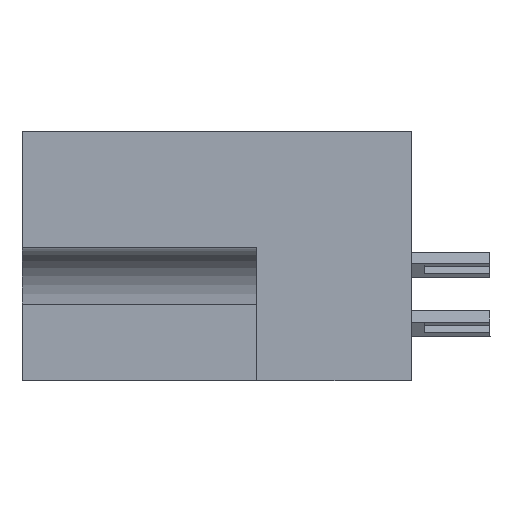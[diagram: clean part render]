
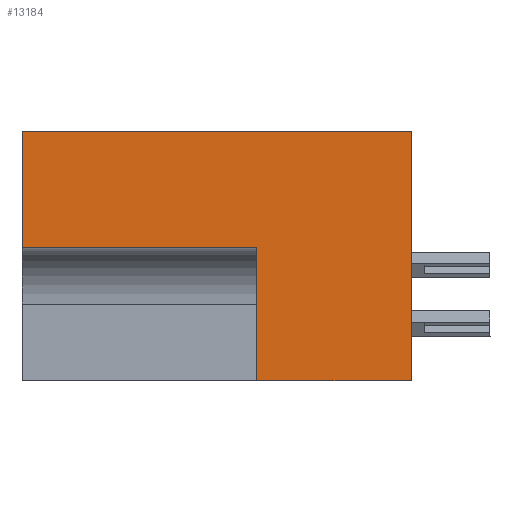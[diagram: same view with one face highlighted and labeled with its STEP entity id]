
A CAD part, left-side view. The second image highlights one B-rep face of the part: STEP entity #13184.
In plain terms, the highlighted planar face has unit normal (-1, 0, 0).
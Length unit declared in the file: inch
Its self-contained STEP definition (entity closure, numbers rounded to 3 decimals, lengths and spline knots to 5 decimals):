
#167 = DIRECTION ( 'NONE',  ( 0., 0., 1. ) ) ;
#720 = LINE ( 'NONE', #21529, #15058 ) ;
#978 = LINE ( 'NONE', #14258, #24172 ) ;
#2013 = EDGE_CURVE ( 'NONE', #28216, #18492, #19542, .T. ) ;
#3158 = CARTESIAN_POINT ( 'NONE',  ( 0., 0., 0. ) ) ;
#3529 = VERTEX_POINT ( 'NONE', #26431 ) ;
#4109 = LINE ( 'NONE', #23786, #12948 ) ;
#4532 = DIRECTION ( 'NONE',  ( 1., 0., 0. ) ) ;
#4587 = AXIS2_PLACEMENT_3D ( 'NONE', #11522, #4532, #9966 ) ;
#5033 = EDGE_CURVE ( 'NONE', #18492, #9611, #13115, .T. ) ;
#6255 = DIRECTION ( 'NONE',  ( 0., -1., 0. ) ) ;
#6435 = EDGE_LOOP ( 'NONE', ( #24551, #23287, #16511, #24964, #24989, #19899 ) ) ;
#9611 = VERTEX_POINT ( 'NONE', #28509 ) ;
#9966 = DIRECTION ( 'NONE',  ( 0., 0., -1. ) ) ;
#10061 = LINE ( 'NONE', #21940, #19622 ) ;
#10692 = VERTEX_POINT ( 'NONE', #24015 ) ;
#11098 = CARTESIAN_POINT ( 'NONE',  ( 0., 0.453, -0.531 ) ) ;
#11186 = CARTESIAN_POINT ( 'NONE',  ( 0., 0., -0.531 ) ) ;
#11245 = CARTESIAN_POINT ( 'NONE',  ( 0., 0.828, 0. ) ) ;
#11522 = CARTESIAN_POINT ( 'NONE',  ( 0., 0.453, 0. ) ) ;
#12258 = EDGE_CURVE ( 'NONE', #28198, #9611, #10061, .T. ) ;
#12635 = DIRECTION ( 'NONE',  ( 0., 0., 1. ) ) ;
#12948 = VECTOR ( 'NONE', #14121, 39.37008 ) ;
#13115 = LINE ( 'NONE', #3158, #20087 ) ;
#13184 = ADVANCED_FACE ( 'NONE', ( #28039 ), #21063, .F. ) ;
#13649 = VECTOR ( 'NONE', #6255, 39.37008 ) ;
#13837 = CARTESIAN_POINT ( 'NONE',  ( 0., 0.328, -0.531 ) ) ;
#14121 = DIRECTION ( 'NONE',  ( 0., 1., 0. ) ) ;
#14258 = CARTESIAN_POINT ( 'NONE',  ( 0., 0.828, 0. ) ) ;
#15058 = VECTOR ( 'NONE', #26176, 39.37008 ) ;
#16455 = EDGE_CURVE ( 'NONE', #10692, #28198, #978, .T. ) ;
#16511 = ORIENTED_EDGE ( 'NONE', *, *, #29806, .F. ) ;
#18492 = VERTEX_POINT ( 'NONE', #11186 ) ;
#19369 = DIRECTION ( 'NONE',  ( 0., -1., 0. ) ) ;
#19542 = LINE ( 'NONE', #11098, #13649 ) ;
#19622 = VECTOR ( 'NONE', #19369, 39.37008 ) ;
#19709 = EDGE_CURVE ( 'NONE', #3529, #10692, #4109, .T. ) ;
#19899 = ORIENTED_EDGE ( 'NONE', *, *, #12258, .F. ) ;
#20087 = VECTOR ( 'NONE', #12635, 39.37008 ) ;
#21063 = PLANE ( 'NONE',  #4587 ) ;
#21529 = CARTESIAN_POINT ( 'NONE',  ( 0., 0.328, -0.531 ) ) ;
#21940 = CARTESIAN_POINT ( 'NONE',  ( 0., 0.453, 0. ) ) ;
#23287 = ORIENTED_EDGE ( 'NONE', *, *, #19709, .F. ) ;
#23786 = CARTESIAN_POINT ( 'NONE',  ( 0., 0.328, -0.248 ) ) ;
#24015 = CARTESIAN_POINT ( 'NONE',  ( 0., 0.828, -0.248 ) ) ;
#24172 = VECTOR ( 'NONE', #167, 39.37008 ) ;
#24551 = ORIENTED_EDGE ( 'NONE', *, *, #16455, .F. ) ;
#24964 = ORIENTED_EDGE ( 'NONE', *, *, #2013, .T. ) ;
#24989 = ORIENTED_EDGE ( 'NONE', *, *, #5033, .T. ) ;
#26176 = DIRECTION ( 'NONE',  ( 0., 0., 1. ) ) ;
#26431 = CARTESIAN_POINT ( 'NONE',  ( 0., 0.328, -0.248 ) ) ;
#28039 = FACE_OUTER_BOUND ( 'NONE', #6435, .T. ) ;
#28198 = VERTEX_POINT ( 'NONE', #11245 ) ;
#28216 = VERTEX_POINT ( 'NONE', #13837 ) ;
#28509 = CARTESIAN_POINT ( 'NONE',  ( 0., 0., 0. ) ) ;
#29806 = EDGE_CURVE ( 'NONE', #28216, #3529, #720, .T. ) ;
